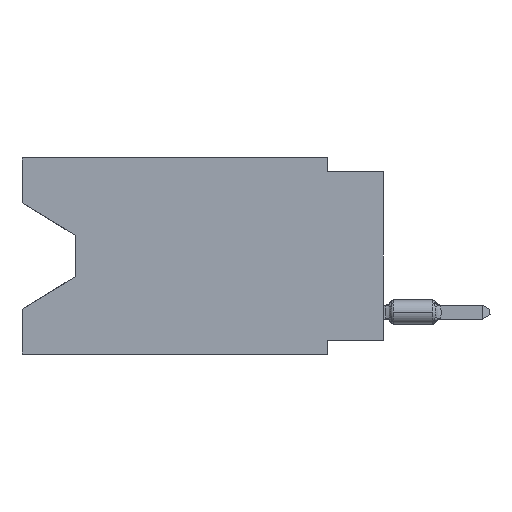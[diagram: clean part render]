
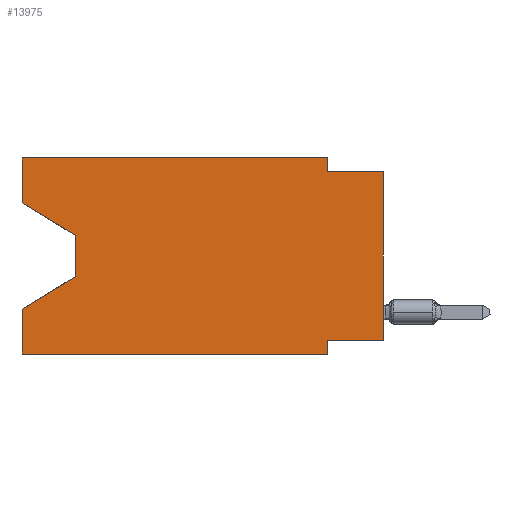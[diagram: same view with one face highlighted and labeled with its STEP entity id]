
A CAD part, left-side view. The second image highlights one B-rep face of the part: STEP entity #13975.
In plain terms, the highlighted planar face has unit normal (-1, 0, 0).
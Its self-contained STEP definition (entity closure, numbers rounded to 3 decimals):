
#358 = CARTESIAN_POINT ( 'NONE',  ( 0., 0., -0.635 ) ) ;
#1017 = VERTEX_POINT ( 'NONE', #27157 ) ;
#1126 = VECTOR ( 'NONE', #27582, 1000. ) ;
#1132 = ORIENTED_EDGE ( 'NONE', *, *, #18474, .T. ) ;
#1355 = CARTESIAN_POINT ( 'NONE',  ( 0., 13.97, -5.385 ) ) ;
#1582 = CARTESIAN_POINT ( 'NONE',  ( 0., 13.97, -5.385 ) ) ;
#2211 = LINE ( 'NONE', #7621, #16028 ) ;
#2318 = LINE ( 'NONE', #13963, #20754 ) ;
#2586 = DIRECTION ( 'NONE',  ( 0., 0., 1. ) ) ;
#3038 = CARTESIAN_POINT ( 'NONE',  ( 0., 16.383, 0. ) ) ;
#3194 = LINE ( 'NONE', #3038, #1126 ) ;
#3272 = DIRECTION ( 'NONE',  ( 0., 0.855, -0.519 ) ) ;
#4227 = ORIENTED_EDGE ( 'NONE', *, *, #26028, .F. ) ;
#4655 = VERTEX_POINT ( 'NONE', #25644 ) ;
#4808 = CARTESIAN_POINT ( 'NONE',  ( 0., 0., -8.255 ) ) ;
#4968 = CARTESIAN_POINT ( 'NONE',  ( 0., 16.383, 0. ) ) ;
#5386 = DIRECTION ( 'NONE',  ( 0., 0., -1. ) ) ;
#6286 = VERTEX_POINT ( 'NONE', #30285 ) ;
#6315 = EDGE_CURVE ( 'NONE', #7923, #11616, #8629, .T. ) ;
#6358 = ORIENTED_EDGE ( 'NONE', *, *, #20044, .T. ) ;
#6472 = CARTESIAN_POINT ( 'NONE',  ( 0., 16.383, 0. ) ) ;
#6548 = CARTESIAN_POINT ( 'NONE',  ( 0., 16.383, 0. ) ) ;
#6643 = AXIS2_PLACEMENT_3D ( 'NONE', #6472, #16188, #25905 ) ;
#7621 = CARTESIAN_POINT ( 'NONE',  ( 0., 16.383, -8.89 ) ) ;
#7855 = EDGE_CURVE ( 'NONE', #13091, #30992, #26704, .T. ) ;
#7923 = VERTEX_POINT ( 'NONE', #29408 ) ;
#8257 = ORIENTED_EDGE ( 'NONE', *, *, #26692, .F. ) ;
#8629 = LINE ( 'NONE', #23416, #20500 ) ;
#8805 = DIRECTION ( 'NONE',  ( 0., 0., -1. ) ) ;
#8828 = CARTESIAN_POINT ( 'NONE',  ( 0., 16.383, -2.038 ) ) ;
#8996 = LINE ( 'NONE', #9472, #9778 ) ;
#9303 = ORIENTED_EDGE ( 'NONE', *, *, #27120, .F. ) ;
#9472 = CARTESIAN_POINT ( 'NONE',  ( 0., 13.97, -3.505 ) ) ;
#9778 = VECTOR ( 'NONE', #28905, 1000. ) ;
#11092 = LINE ( 'NONE', #1355, #28848 ) ;
#11275 = FACE_OUTER_BOUND ( 'NONE', #25071, .T. ) ;
#11360 = ORIENTED_EDGE ( 'NONE', *, *, #6315, .F. ) ;
#11482 = VECTOR ( 'NONE', #8805, 1000. ) ;
#11616 = VERTEX_POINT ( 'NONE', #13530 ) ;
#12810 = CARTESIAN_POINT ( 'NONE',  ( 0., 16.383, -2.038 ) ) ;
#12992 = VERTEX_POINT ( 'NONE', #21207 ) ;
#13091 = VERTEX_POINT ( 'NONE', #13105 ) ;
#13105 = CARTESIAN_POINT ( 'NONE',  ( 0., 2.54, -0.635 ) ) ;
#13481 = ORIENTED_EDGE ( 'NONE', *, *, #16510, .F. ) ;
#13530 = CARTESIAN_POINT ( 'NONE',  ( 0., 16.383, -6.852 ) ) ;
#13963 = CARTESIAN_POINT ( 'NONE',  ( 0., 0., 0. ) ) ;
#13975 = ADVANCED_FACE ( 'NONE', ( #11275 ), #28294, .F. ) ;
#14223 = ORIENTED_EDGE ( 'NONE', *, *, #31499, .F. ) ;
#14535 = DIRECTION ( 'NONE',  ( 0., 1., 0. ) ) ;
#14725 = VERTEX_POINT ( 'NONE', #1582 ) ;
#15365 = DIRECTION ( 'NONE',  ( 0., -0.855, -0.519 ) ) ;
#16028 = VECTOR ( 'NONE', #29282, 1000. ) ;
#16188 = DIRECTION ( 'NONE',  ( 1., 0., 0. ) ) ;
#16207 = EDGE_CURVE ( 'NONE', #17689, #12992, #23143, .T. ) ;
#16508 = DIRECTION ( 'NONE',  ( 0., 0., 1. ) ) ;
#16510 = EDGE_CURVE ( 'NONE', #17689, #27385, #27118, .T. ) ;
#16892 = CARTESIAN_POINT ( 'NONE',  ( 0., 0., -8.255 ) ) ;
#17305 = VECTOR ( 'NONE', #15365, 1000. ) ;
#17689 = VERTEX_POINT ( 'NONE', #12810 ) ;
#18318 = DIRECTION ( 'NONE',  ( 0., 0., 1. ) ) ;
#18474 = EDGE_CURVE ( 'NONE', #14725, #11616, #11092, .T. ) ;
#19054 = CARTESIAN_POINT ( 'NONE',  ( 0., 0., -0.635 ) ) ;
#19939 = ORIENTED_EDGE ( 'NONE', *, *, #16207, .T. ) ;
#20044 = EDGE_CURVE ( 'NONE', #7923, #4655, #2211, .T. ) ;
#20500 = VECTOR ( 'NONE', #18318, 1000. ) ;
#20754 = VECTOR ( 'NONE', #16508, 1000. ) ;
#21051 = ORIENTED_EDGE ( 'NONE', *, *, #7855, .F. ) ;
#21207 = CARTESIAN_POINT ( 'NONE',  ( 0., 13.97, -3.505 ) ) ;
#21414 = VECTOR ( 'NONE', #2586, 1000. ) ;
#21644 = CARTESIAN_POINT ( 'NONE',  ( 0., 2.54, 0. ) ) ;
#21973 = LINE ( 'NONE', #21644, #25220 ) ;
#22329 = VECTOR ( 'NONE', #26229, 1000. ) ;
#22980 = CARTESIAN_POINT ( 'NONE',  ( 0., 2.54, -8.89 ) ) ;
#23143 = LINE ( 'NONE', #8828, #17305 ) ;
#23416 = CARTESIAN_POINT ( 'NONE',  ( 0., 16.383, 0. ) ) ;
#24101 = EDGE_CURVE ( 'NONE', #27459, #30992, #2318, .T. ) ;
#24917 = ORIENTED_EDGE ( 'NONE', *, *, #24101, .T. ) ;
#25053 = LINE ( 'NONE', #22980, #11482 ) ;
#25071 = EDGE_LOOP ( 'NONE', ( #19939, #28932, #1132, #11360, #6358, #4227, #9303, #24917, #21051, #8257, #14223, #13481 ) ) ;
#25220 = VECTOR ( 'NONE', #5386, 1000. ) ;
#25644 = CARTESIAN_POINT ( 'NONE',  ( 0., 2.54, -8.89 ) ) ;
#25905 = DIRECTION ( 'NONE',  ( 0., 0., -1. ) ) ;
#26028 = EDGE_CURVE ( 'NONE', #6286, #4655, #25053, .T. ) ;
#26229 = DIRECTION ( 'NONE',  ( 0., -1., 0. ) ) ;
#26647 = LINE ( 'NONE', #4808, #27891 ) ;
#26692 = EDGE_CURVE ( 'NONE', #1017, #13091, #21973, .T. ) ;
#26704 = LINE ( 'NONE', #19054, #22329 ) ;
#27118 = LINE ( 'NONE', #4968, #21414 ) ;
#27120 = EDGE_CURVE ( 'NONE', #27459, #6286, #26647, .T. ) ;
#27157 = CARTESIAN_POINT ( 'NONE',  ( 0., 2.54, 0. ) ) ;
#27385 = VERTEX_POINT ( 'NONE', #6548 ) ;
#27459 = VERTEX_POINT ( 'NONE', #16892 ) ;
#27582 = DIRECTION ( 'NONE',  ( 0., -1., 0. ) ) ;
#27891 = VECTOR ( 'NONE', #14535, 1000. ) ;
#28294 = PLANE ( 'NONE',  #6643 ) ;
#28848 = VECTOR ( 'NONE', #3272, 1000. ) ;
#28905 = DIRECTION ( 'NONE',  ( 0., 0., -1. ) ) ;
#28932 = ORIENTED_EDGE ( 'NONE', *, *, #30835, .T. ) ;
#29282 = DIRECTION ( 'NONE',  ( 0., -1., 0. ) ) ;
#29408 = CARTESIAN_POINT ( 'NONE',  ( 0., 16.383, -8.89 ) ) ;
#30285 = CARTESIAN_POINT ( 'NONE',  ( 0., 2.54, -8.255 ) ) ;
#30835 = EDGE_CURVE ( 'NONE', #12992, #14725, #8996, .T. ) ;
#30992 = VERTEX_POINT ( 'NONE', #358 ) ;
#31499 = EDGE_CURVE ( 'NONE', #27385, #1017, #3194, .T. ) ;
